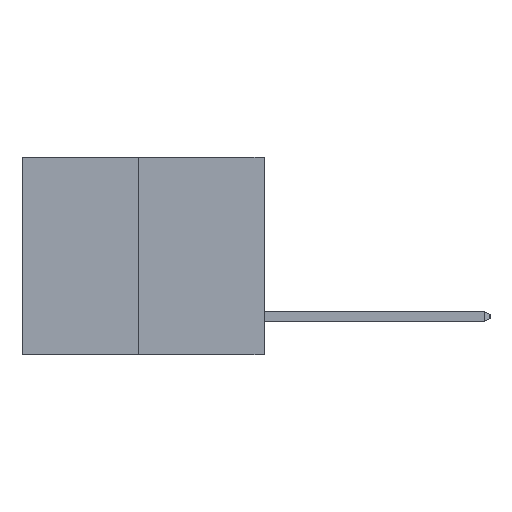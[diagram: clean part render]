
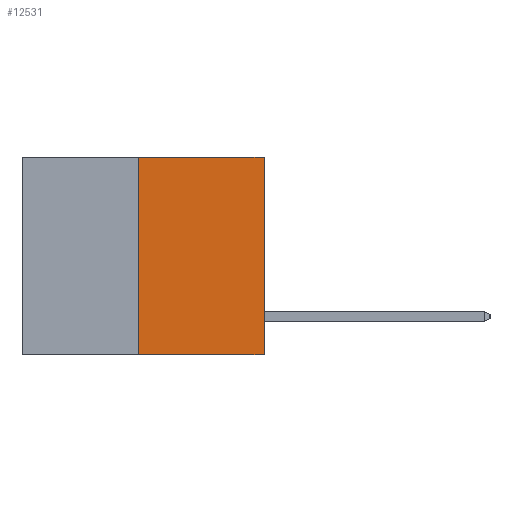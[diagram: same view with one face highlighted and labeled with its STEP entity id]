
A CAD part, left-side view. The second image highlights one B-rep face of the part: STEP entity #12531.
In plain terms, the highlighted planar face has unit normal (-1, 0, 0).
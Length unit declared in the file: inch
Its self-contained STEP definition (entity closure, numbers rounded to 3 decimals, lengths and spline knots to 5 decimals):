
#481 = LINE ( 'NONE', #24157, #21480 ) ;
#675 = EDGE_CURVE ( 'NONE', #21204, #8818, #14201, .T. ) ;
#1181 = CARTESIAN_POINT ( 'NONE',  ( 0., 0., 0. ) ) ;
#1579 = CARTESIAN_POINT ( 'NONE',  ( 0., 0., 0. ) ) ;
#1854 = VECTOR ( 'NONE', #6824, 39.37008 ) ;
#3097 = LINE ( 'NONE', #21284, #1854 ) ;
#4289 = ORIENTED_EDGE ( 'NONE', *, *, #14637, .F. ) ;
#5067 = CARTESIAN_POINT ( 'NONE',  ( 0., 0.312, -0.49 ) ) ;
#6726 = EDGE_CURVE ( 'NONE', #8818, #12037, #25045, .T. ) ;
#6824 = DIRECTION ( 'NONE',  ( 0., 0., 1. ) ) ;
#7149 = AXIS2_PLACEMENT_3D ( 'NONE', #12370, #10204, #7804 ) ;
#7167 = CARTESIAN_POINT ( 'NONE',  ( 0., 0., -0.49 ) ) ;
#7804 = DIRECTION ( 'NONE',  ( 0., 0., -1. ) ) ;
#8084 = EDGE_CURVE ( 'NONE', #18634, #12037, #481, .T. ) ;
#8818 = VERTEX_POINT ( 'NONE', #7167 ) ;
#10204 = DIRECTION ( 'NONE',  ( 1., 0., 0. ) ) ;
#11896 = CARTESIAN_POINT ( 'NONE',  ( 0., 0.6, -0.49 ) ) ;
#11975 = DIRECTION ( 'NONE',  ( 0., -1., 0. ) ) ;
#12037 = VERTEX_POINT ( 'NONE', #1579 ) ;
#12370 = CARTESIAN_POINT ( 'NONE',  ( 0., 0.6, 0. ) ) ;
#12531 = ADVANCED_FACE ( 'NONE', ( #20699 ), #18435, .F. ) ;
#13305 = ORIENTED_EDGE ( 'NONE', *, *, #8084, .F. ) ;
#14190 = VECTOR ( 'NONE', #23166, 39.37008 ) ;
#14201 = LINE ( 'NONE', #11896, #25699 ) ;
#14637 = EDGE_CURVE ( 'NONE', #21204, #18634, #3097, .T. ) ;
#16220 = DIRECTION ( 'NONE',  ( 0., -1., 0. ) ) ;
#16535 = EDGE_LOOP ( 'NONE', ( #4289, #24535, #16701, #13305 ) ) ;
#16701 = ORIENTED_EDGE ( 'NONE', *, *, #6726, .T. ) ;
#18435 = PLANE ( 'NONE',  #7149 ) ;
#18634 = VERTEX_POINT ( 'NONE', #18970 ) ;
#18970 = CARTESIAN_POINT ( 'NONE',  ( 0., 0.312, 0. ) ) ;
#20699 = FACE_OUTER_BOUND ( 'NONE', #16535, .T. ) ;
#21204 = VERTEX_POINT ( 'NONE', #5067 ) ;
#21284 = CARTESIAN_POINT ( 'NONE',  ( 0., 0.312, -0.49 ) ) ;
#21480 = VECTOR ( 'NONE', #11975, 39.37008 ) ;
#23166 = DIRECTION ( 'NONE',  ( 0., 0., 1. ) ) ;
#24157 = CARTESIAN_POINT ( 'NONE',  ( 0., 0.6, 0. ) ) ;
#24535 = ORIENTED_EDGE ( 'NONE', *, *, #675, .T. ) ;
#25045 = LINE ( 'NONE', #1181, #14190 ) ;
#25699 = VECTOR ( 'NONE', #16220, 39.37008 ) ;
